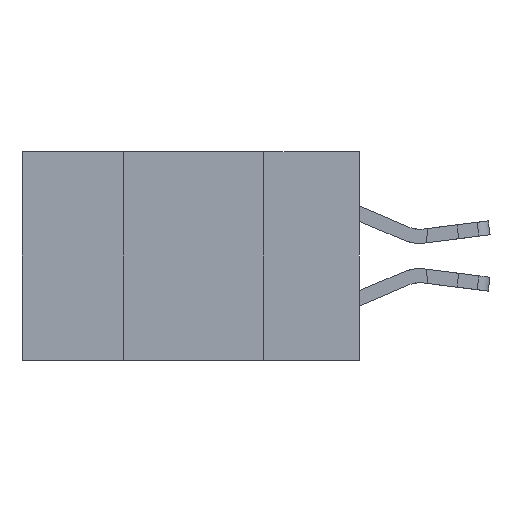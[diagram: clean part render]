
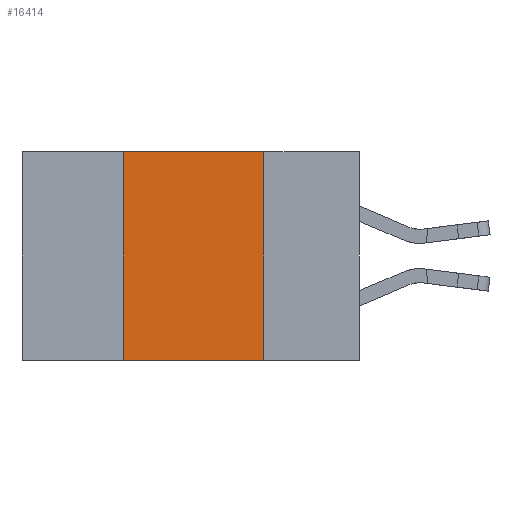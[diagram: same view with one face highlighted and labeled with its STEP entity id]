
A CAD part, left-side view. The second image highlights one B-rep face of the part: STEP entity #16414.
In plain terms, the highlighted planar face has unit normal (-1, 0, 0).
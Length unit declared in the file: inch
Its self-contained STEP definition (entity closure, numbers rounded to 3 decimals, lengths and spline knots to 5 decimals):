
#997 = LINE ( 'NONE', #12920, #7125 ) ;
#1231 = LINE ( 'NONE', #9340, #17647 ) ;
#3038 = CARTESIAN_POINT ( 'NONE',  ( 0., 0.17, 0. ) ) ;
#3462 = EDGE_CURVE ( 'NONE', #14113, #4862, #1231, .T. ) ;
#3785 = LINE ( 'NONE', #4468, #22161 ) ;
#4468 = CARTESIAN_POINT ( 'NONE',  ( 0., 0.42, 0. ) ) ;
#4862 = VERTEX_POINT ( 'NONE', #21662 ) ;
#5078 = VERTEX_POINT ( 'NONE', #5558 ) ;
#5558 = CARTESIAN_POINT ( 'NONE',  ( 0., 0.17, -0.37 ) ) ;
#7125 = VECTOR ( 'NONE', #16448, 39.37008 ) ;
#8396 = LINE ( 'NONE', #3038, #13698 ) ;
#8719 = VERTEX_POINT ( 'NONE', #10712 ) ;
#9340 = CARTESIAN_POINT ( 'NONE',  ( 0., 0.6, 0. ) ) ;
#10712 = CARTESIAN_POINT ( 'NONE',  ( 0., 0.42, -0.37 ) ) ;
#11007 = AXIS2_PLACEMENT_3D ( 'NONE', #18358, #17176, #13477 ) ;
#12773 = FACE_OUTER_BOUND ( 'NONE', #18521, .T. ) ;
#12920 = CARTESIAN_POINT ( 'NONE',  ( 0., 0.6, -0.37 ) ) ;
#13424 = DIRECTION ( 'NONE',  ( 0., 0., 1. ) ) ;
#13477 = DIRECTION ( 'NONE',  ( 0., 0., -1. ) ) ;
#13698 = VECTOR ( 'NONE', #22641, 39.37008 ) ;
#14113 = VERTEX_POINT ( 'NONE', #18254 ) ;
#16235 = ORIENTED_EDGE ( 'NONE', *, *, #22797, .F. ) ;
#16414 = ADVANCED_FACE ( 'NONE', ( #12773 ), #16562, .F. ) ;
#16448 = DIRECTION ( 'NONE',  ( 0., -1., 0. ) ) ;
#16562 = PLANE ( 'NONE',  #11007 ) ;
#17176 = DIRECTION ( 'NONE',  ( 1., 0., 0. ) ) ;
#17415 = EDGE_CURVE ( 'NONE', #8719, #14113, #3785, .T. ) ;
#17647 = VECTOR ( 'NONE', #21012, 39.37008 ) ;
#18254 = CARTESIAN_POINT ( 'NONE',  ( 0., 0.42, 0. ) ) ;
#18276 = ORIENTED_EDGE ( 'NONE', *, *, #20177, .T. ) ;
#18358 = CARTESIAN_POINT ( 'NONE',  ( 0., 0.6, 0. ) ) ;
#18521 = EDGE_LOOP ( 'NONE', ( #16235, #20703, #20140, #18276 ) ) ;
#20140 = ORIENTED_EDGE ( 'NONE', *, *, #17415, .F. ) ;
#20177 = EDGE_CURVE ( 'NONE', #8719, #5078, #997, .T. ) ;
#20703 = ORIENTED_EDGE ( 'NONE', *, *, #3462, .F. ) ;
#21012 = DIRECTION ( 'NONE',  ( 0., -1., 0. ) ) ;
#21662 = CARTESIAN_POINT ( 'NONE',  ( 0., 0.17, 0. ) ) ;
#22161 = VECTOR ( 'NONE', #13424, 39.37008 ) ;
#22641 = DIRECTION ( 'NONE',  ( 0., 0., -1. ) ) ;
#22797 = EDGE_CURVE ( 'NONE', #4862, #5078, #8396, .T. ) ;
